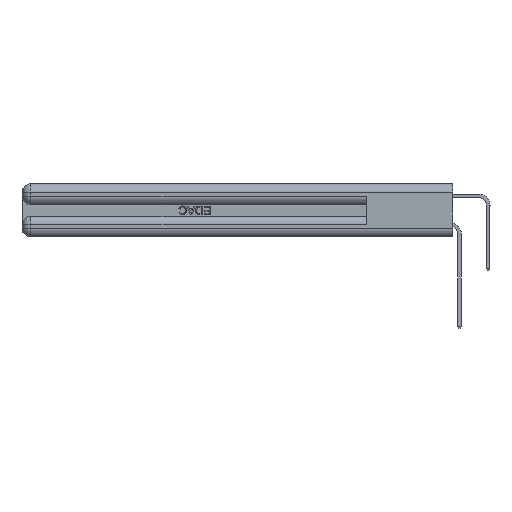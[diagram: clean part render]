
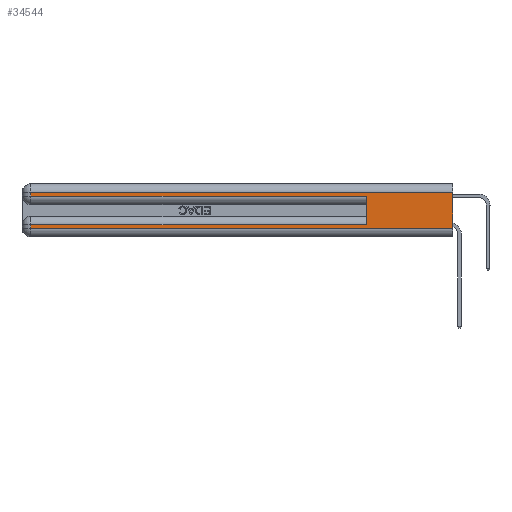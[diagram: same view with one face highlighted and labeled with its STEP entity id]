
A CAD part, left-side view. The second image highlights one B-rep face of the part: STEP entity #34544.
In plain terms, the highlighted planar face has unit normal (-1, 0, 0).
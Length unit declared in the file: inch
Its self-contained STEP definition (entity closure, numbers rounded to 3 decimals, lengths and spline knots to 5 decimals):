
#203 = VERTEX_POINT ( 'NONE', #32718 ) ;
#525 = PLANE ( 'NONE',  #18624 ) ;
#545 = LINE ( 'NONE', #27678, #22072 ) ;
#757 = CARTESIAN_POINT ( 'NONE',  ( 0., 2.94, 0.06 ) ) ;
#1581 = CARTESIAN_POINT ( 'NONE',  ( 0., 2.94, 0.31 ) ) ;
#2519 = EDGE_CURVE ( 'NONE', #21736, #43947, #2544, .T. ) ;
#2544 = LINE ( 'NONE', #11573, #44467 ) ;
#2621 = EDGE_CURVE ( 'NONE', #46712, #13871, #11552, .T. ) ;
#2856 = FACE_OUTER_BOUND ( 'NONE', #9499, .T. ) ;
#3717 = ORIENTED_EDGE ( 'NONE', *, *, #41786, .T. ) ;
#3967 = VECTOR ( 'NONE', #17713, 39.37008 ) ;
#4308 = LINE ( 'NONE', #5109, #18047 ) ;
#5109 = CARTESIAN_POINT ( 'NONE',  ( 0., 2.94, 0.37 ) ) ;
#6972 = CARTESIAN_POINT ( 'NONE',  ( 0., 2.94, 0.37 ) ) ;
#8646 = DIRECTION ( 'NONE',  ( 0., -1., 0. ) ) ;
#8939 = DIRECTION ( 'NONE',  ( 0., 0., -1. ) ) ;
#8995 = CARTESIAN_POINT ( 'NONE',  ( 0., 0.6, 0.285 ) ) ;
#9499 = EDGE_LOOP ( 'NONE', ( #30069, #42074, #43231, #41449, #32420, #3717, #38310, #24104 ) ) ;
#9798 = VERTEX_POINT ( 'NONE', #27394 ) ;
#10207 = EDGE_CURVE ( 'NONE', #46712, #37847, #34863, .T. ) ;
#10223 = VECTOR ( 'NONE', #41638, 39.37008 ) ;
#10522 = VERTEX_POINT ( 'NONE', #757 ) ;
#11552 = LINE ( 'NONE', #31600, #28250 ) ;
#11573 = CARTESIAN_POINT ( 'NONE',  ( 0., 0.6, 0.145 ) ) ;
#12625 = VECTOR ( 'NONE', #45118, 39.37008 ) ;
#13871 = VERTEX_POINT ( 'NONE', #24116 ) ;
#15760 = DIRECTION ( 'NONE',  ( 1., 0., 0. ) ) ;
#17523 = VECTOR ( 'NONE', #17864, 39.37008 ) ;
#17713 = DIRECTION ( 'NONE',  ( 0., 1., 0. ) ) ;
#17864 = DIRECTION ( 'NONE',  ( 0., 1., 0. ) ) ;
#18047 = VECTOR ( 'NONE', #8939, 39.37008 ) ;
#18624 = AXIS2_PLACEMENT_3D ( 'NONE', #27090, #15760, #23267 ) ;
#21736 = VERTEX_POINT ( 'NONE', #26754 ) ;
#22072 = VECTOR ( 'NONE', #8646, 39.37008 ) ;
#23267 = DIRECTION ( 'NONE',  ( 0., 0., -1. ) ) ;
#24104 = ORIENTED_EDGE ( 'NONE', *, *, #28835, .T. ) ;
#24116 = CARTESIAN_POINT ( 'NONE',  ( 0., 0., 0.06 ) ) ;
#26754 = CARTESIAN_POINT ( 'NONE',  ( 0., 0.6, 0.085 ) ) ;
#27090 = CARTESIAN_POINT ( 'NONE',  ( 0., 0., 0.37 ) ) ;
#27394 = CARTESIAN_POINT ( 'NONE',  ( 0., 2.94, 0.085 ) ) ;
#27678 = CARTESIAN_POINT ( 'NONE',  ( 0., 0., 0.285 ) ) ;
#27762 = EDGE_CURVE ( 'NONE', #37847, #203, #4308, .T. ) ;
#28250 = VECTOR ( 'NONE', #31256, 39.37008 ) ;
#28835 = EDGE_CURVE ( 'NONE', #10522, #13871, #30560, .T. ) ;
#30069 = ORIENTED_EDGE ( 'NONE', *, *, #2621, .F. ) ;
#30560 = LINE ( 'NONE', #41469, #10223 ) ;
#31256 = DIRECTION ( 'NONE',  ( 0., 0., -1. ) ) ;
#31600 = CARTESIAN_POINT ( 'NONE',  ( 0., 0., 0.37 ) ) ;
#32420 = ORIENTED_EDGE ( 'NONE', *, *, #2519, .F. ) ;
#32718 = CARTESIAN_POINT ( 'NONE',  ( 0., 2.94, 0.285 ) ) ;
#34544 = ADVANCED_FACE ( 'NONE', ( #2856 ), #525, .F. ) ;
#34753 = LINE ( 'NONE', #6972, #12625 ) ;
#34863 = LINE ( 'NONE', #36909, #17523 ) ;
#36909 = CARTESIAN_POINT ( 'NONE',  ( 0., 0., 0.31 ) ) ;
#37847 = VERTEX_POINT ( 'NONE', #1581 ) ;
#38310 = ORIENTED_EDGE ( 'NONE', *, *, #44057, .T. ) ;
#40266 = EDGE_CURVE ( 'NONE', #203, #43947, #545, .T. ) ;
#40604 = CARTESIAN_POINT ( 'NONE',  ( 0., 0., 0.085 ) ) ;
#41449 = ORIENTED_EDGE ( 'NONE', *, *, #40266, .T. ) ;
#41469 = CARTESIAN_POINT ( 'NONE',  ( 0., 0., 0.06 ) ) ;
#41511 = DIRECTION ( 'NONE',  ( 0., 0., 1. ) ) ;
#41638 = DIRECTION ( 'NONE',  ( 0., -1., 0. ) ) ;
#41693 = LINE ( 'NONE', #40604, #3967 ) ;
#41786 = EDGE_CURVE ( 'NONE', #21736, #9798, #41693, .T. ) ;
#42074 = ORIENTED_EDGE ( 'NONE', *, *, #10207, .T. ) ;
#43231 = ORIENTED_EDGE ( 'NONE', *, *, #27762, .T. ) ;
#43947 = VERTEX_POINT ( 'NONE', #8995 ) ;
#44057 = EDGE_CURVE ( 'NONE', #9798, #10522, #34753, .T. ) ;
#44467 = VECTOR ( 'NONE', #41511, 39.37008 ) ;
#45118 = DIRECTION ( 'NONE',  ( 0., 0., -1. ) ) ;
#46712 = VERTEX_POINT ( 'NONE', #48112 ) ;
#48112 = CARTESIAN_POINT ( 'NONE',  ( 0., 0., 0.31 ) ) ;
